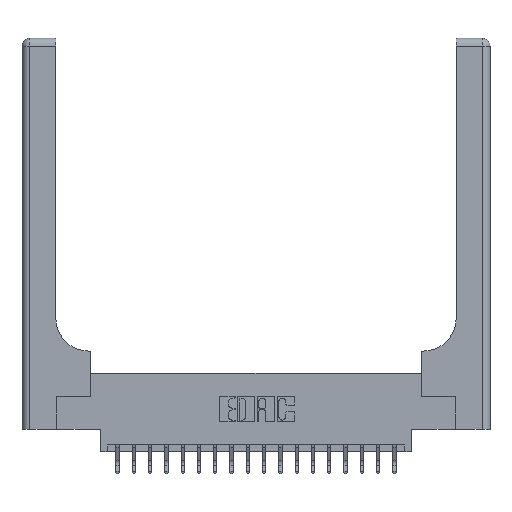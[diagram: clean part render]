
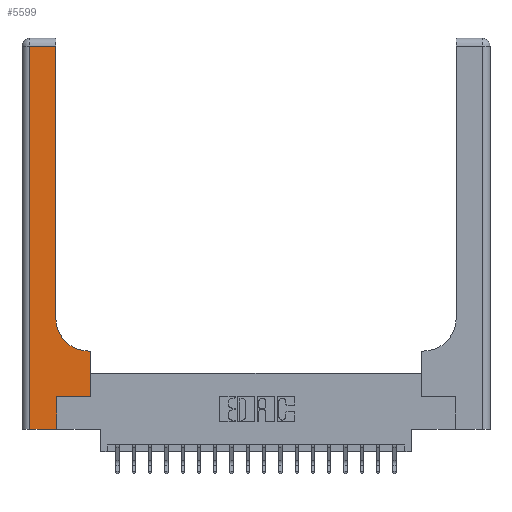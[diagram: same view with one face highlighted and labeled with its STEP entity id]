
A CAD part, top view. The second image highlights one B-rep face of the part: STEP entity #5599.
In plain terms, the highlighted planar face has unit normal (0, 0, 1).
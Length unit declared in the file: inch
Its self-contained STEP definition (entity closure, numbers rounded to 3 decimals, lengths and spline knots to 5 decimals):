
#525 = CIRCLE ( 'NONE', #11737, 0.25 ) ;
#1252 = CARTESIAN_POINT ( 'NONE',  ( 0.51, 0.6, 0.37 ) ) ;
#1294 = VERTEX_POINT ( 'NONE', #1252 ) ;
#1507 = CARTESIAN_POINT ( 'NONE',  ( 0.06, 2.94, 0.37 ) ) ;
#2074 = DIRECTION ( 'NONE',  ( -1., 0., 0. ) ) ;
#2697 = VECTOR ( 'NONE', #19187, 39.37008 ) ;
#2819 = EDGE_CURVE ( 'NONE', #5847, #14470, #9841, .T. ) ;
#2863 = LINE ( 'NONE', #9625, #6845 ) ;
#3416 = VECTOR ( 'NONE', #5402, 39.37008 ) ;
#4617 = CARTESIAN_POINT ( 'NONE',  ( 0.265, 0., 0.37 ) ) ;
#4794 = VERTEX_POINT ( 'NONE', #8057 ) ;
#5081 = ORIENTED_EDGE ( 'NONE', *, *, #8814, .T. ) ;
#5098 = DIRECTION ( 'NONE',  ( 0., 1., 0. ) ) ;
#5144 = CARTESIAN_POINT ( 'NONE',  ( 0., 3., 0.37 ) ) ;
#5402 = DIRECTION ( 'NONE',  ( 0., 1., 0. ) ) ;
#5503 = CARTESIAN_POINT ( 'NONE',  ( 0.528, 0.25, 0.37 ) ) ;
#5599 = ADVANCED_FACE ( 'NONE', ( #19449 ), #19764, .F. ) ;
#5847 = VERTEX_POINT ( 'NONE', #8734 ) ;
#6621 = CARTESIAN_POINT ( 'NONE',  ( 0.26, 3., 0.37 ) ) ;
#6845 = VECTOR ( 'NONE', #16080, 39.37008 ) ;
#6923 = ORIENTED_EDGE ( 'NONE', *, *, #18920, .T. ) ;
#7217 = LINE ( 'NONE', #13491, #16935 ) ;
#7416 = DIRECTION ( 'NONE',  ( 1., 0., 0. ) ) ;
#7485 = CARTESIAN_POINT ( 'NONE',  ( 0.265, 0.25, 0.37 ) ) ;
#7886 = EDGE_CURVE ( 'NONE', #16263, #1294, #2863, .T. ) ;
#7937 = DIRECTION ( 'NONE',  ( 0., 1., 0. ) ) ;
#8057 = CARTESIAN_POINT ( 'NONE',  ( 0.265, 0.25, 0.37 ) ) ;
#8734 = CARTESIAN_POINT ( 'NONE',  ( 0.26, 0.85, 0.37 ) ) ;
#8754 = VERTEX_POINT ( 'NONE', #4617 ) ;
#8814 = EDGE_CURVE ( 'NONE', #4794, #11455, #10709, .T. ) ;
#9023 = CARTESIAN_POINT ( 'NONE',  ( 0.528, 0.6, 0.37 ) ) ;
#9252 = ORIENTED_EDGE ( 'NONE', *, *, #20586, .T. ) ;
#9625 = CARTESIAN_POINT ( 'NONE',  ( 0.26, 0.6, 0.37 ) ) ;
#9841 = LINE ( 'NONE', #6621, #15846 ) ;
#9954 = VECTOR ( 'NONE', #13953, 39.37008 ) ;
#10129 = ORIENTED_EDGE ( 'NONE', *, *, #16445, .T. ) ;
#10709 = LINE ( 'NONE', #7485, #9954 ) ;
#10793 = EDGE_CURVE ( 'NONE', #18185, #16941, #20402, .T. ) ;
#10795 = VECTOR ( 'NONE', #5098, 39.37008 ) ;
#10948 = LINE ( 'NONE', #12532, #2697 ) ;
#11118 = DIRECTION ( 'NONE',  ( 1., 0., 0. ) ) ;
#11455 = VERTEX_POINT ( 'NONE', #13687 ) ;
#11670 = ORIENTED_EDGE ( 'NONE', *, *, #7886, .T. ) ;
#11737 = AXIS2_PLACEMENT_3D ( 'NONE', #17234, #17339, #11118 ) ;
#12176 = CARTESIAN_POINT ( 'NONE',  ( 0.06, 3., 0.37 ) ) ;
#12310 = LINE ( 'NONE', #5503, #3416 ) ;
#12532 = CARTESIAN_POINT ( 'NONE',  ( 0., 2.94, 0.37 ) ) ;
#12837 = ORIENTED_EDGE ( 'NONE', *, *, #10793, .T. ) ;
#13224 = EDGE_CURVE ( 'NONE', #1294, #5847, #525, .T. ) ;
#13491 = CARTESIAN_POINT ( 'NONE',  ( 0., 0., 0.37 ) ) ;
#13687 = CARTESIAN_POINT ( 'NONE',  ( 0.528, 0.25, 0.37 ) ) ;
#13953 = DIRECTION ( 'NONE',  ( 1., 0., 0. ) ) ;
#14470 = VERTEX_POINT ( 'NONE', #19141 ) ;
#14721 = VECTOR ( 'NONE', #15635, 39.37008 ) ;
#14865 = EDGE_LOOP ( 'NONE', ( #16666, #10129, #12837, #6923, #16123, #5081, #9252, #11670, #20239 ) ) ;
#15449 = EDGE_CURVE ( 'NONE', #8754, #4794, #18030, .T. ) ;
#15635 = DIRECTION ( 'NONE',  ( 0., -1., 0. ) ) ;
#15777 = AXIS2_PLACEMENT_3D ( 'NONE', #5144, #16700, #2074 ) ;
#15846 = VECTOR ( 'NONE', #7937, 39.37008 ) ;
#16080 = DIRECTION ( 'NONE',  ( -1., 0., 0. ) ) ;
#16123 = ORIENTED_EDGE ( 'NONE', *, *, #15449, .T. ) ;
#16263 = VERTEX_POINT ( 'NONE', #9023 ) ;
#16445 = EDGE_CURVE ( 'NONE', #14470, #18185, #10948, .T. ) ;
#16666 = ORIENTED_EDGE ( 'NONE', *, *, #2819, .T. ) ;
#16700 = DIRECTION ( 'NONE',  ( 0., 0., -1. ) ) ;
#16935 = VECTOR ( 'NONE', #7416, 39.37008 ) ;
#16941 = VERTEX_POINT ( 'NONE', #19645 ) ;
#17234 = CARTESIAN_POINT ( 'NONE',  ( 0.51, 0.85, 0.37 ) ) ;
#17339 = DIRECTION ( 'NONE',  ( 0., 0., -1. ) ) ;
#18030 = LINE ( 'NONE', #18353, #10795 ) ;
#18185 = VERTEX_POINT ( 'NONE', #1507 ) ;
#18353 = CARTESIAN_POINT ( 'NONE',  ( 0.265, 0., 0.37 ) ) ;
#18920 = EDGE_CURVE ( 'NONE', #16941, #8754, #7217, .T. ) ;
#19141 = CARTESIAN_POINT ( 'NONE',  ( 0.26, 2.94, 0.37 ) ) ;
#19187 = DIRECTION ( 'NONE',  ( -1., 0., 0. ) ) ;
#19449 = FACE_OUTER_BOUND ( 'NONE', #14865, .T. ) ;
#19645 = CARTESIAN_POINT ( 'NONE',  ( 0.06, 0., 0.37 ) ) ;
#19764 = PLANE ( 'NONE',  #15777 ) ;
#20239 = ORIENTED_EDGE ( 'NONE', *, *, #13224, .T. ) ;
#20402 = LINE ( 'NONE', #12176, #14721 ) ;
#20586 = EDGE_CURVE ( 'NONE', #11455, #16263, #12310, .T. ) ;
